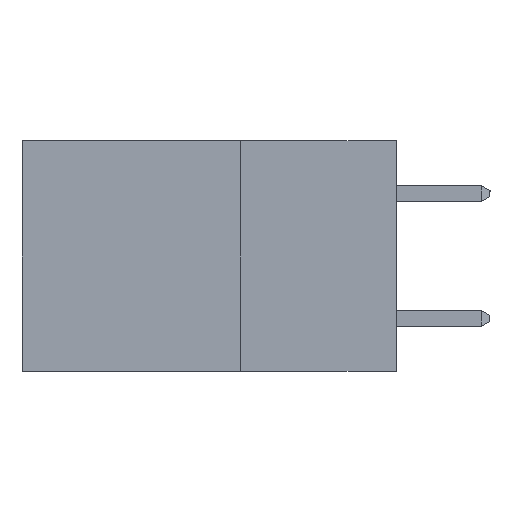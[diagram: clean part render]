
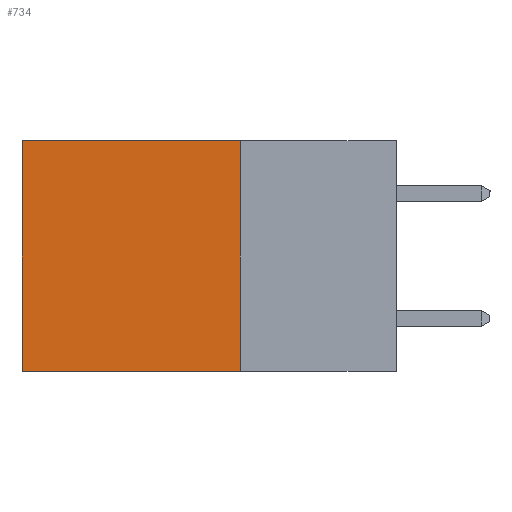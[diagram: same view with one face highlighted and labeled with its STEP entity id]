
A CAD part, left-side view. The second image highlights one B-rep face of the part: STEP entity #734.
In plain terms, the highlighted planar face has unit normal (-1, 0, 0).
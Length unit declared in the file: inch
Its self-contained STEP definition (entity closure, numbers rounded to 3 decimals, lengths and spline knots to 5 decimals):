
#233 = ORIENTED_EDGE ( 'NONE', *, *, #7456, .F. ) ;
#541 = DIRECTION ( 'NONE',  ( 1., 0., 0. ) ) ;
#602 = CARTESIAN_POINT ( 'NONE',  ( 0.2615, 0.6, -0.37 ) ) ;
#645 = CARTESIAN_POINT ( 'NONE',  ( 0.2615, 0.25, 0. ) ) ;
#662 = LINE ( 'NONE', #11323, #1744 ) ;
#734 = ADVANCED_FACE ( 'NONE', ( #12336 ), #2874, .F. ) ;
#1647 = ORIENTED_EDGE ( 'NONE', *, *, #8013, .T. ) ;
#1744 = VECTOR ( 'NONE', #6062, 39.37008 ) ;
#2865 = VECTOR ( 'NONE', #16594, 39.37008 ) ;
#2874 = PLANE ( 'NONE',  #13465 ) ;
#3467 = ORIENTED_EDGE ( 'NONE', *, *, #10542, .T. ) ;
#4374 = CARTESIAN_POINT ( 'NONE',  ( 0.2615, 0.25, -0.37 ) ) ;
#6062 = DIRECTION ( 'NONE',  ( 0., 1., 0. ) ) ;
#6127 = DIRECTION ( 'NONE',  ( 0., 0., -1. ) ) ;
#6143 = CARTESIAN_POINT ( 'NONE',  ( 0.2615, 0.6, -0.37 ) ) ;
#7348 = VERTEX_POINT ( 'NONE', #645 ) ;
#7456 = EDGE_CURVE ( 'NONE', #7348, #13316, #9012, .T. ) ;
#8013 = EDGE_CURVE ( 'NONE', #7348, #10789, #662, .T. ) ;
#8513 = LINE ( 'NONE', #6143, #2865 ) ;
#9012 = LINE ( 'NONE', #10422, #16290 ) ;
#9901 = DIRECTION ( 'NONE',  ( 0., 0., -1. ) ) ;
#10422 = CARTESIAN_POINT ( 'NONE',  ( 0.2615, 0.25, -0.37 ) ) ;
#10542 = EDGE_CURVE ( 'NONE', #10789, #15559, #8513, .T. ) ;
#10789 = VERTEX_POINT ( 'NONE', #12084 ) ;
#10847 = EDGE_LOOP ( 'NONE', ( #3467, #14903, #233, #1647 ) ) ;
#11285 = DIRECTION ( 'NONE',  ( 0., 1., 0. ) ) ;
#11323 = CARTESIAN_POINT ( 'NONE',  ( 0.2615, 0.25, 0. ) ) ;
#12084 = CARTESIAN_POINT ( 'NONE',  ( 0.2615, 0.6, 0. ) ) ;
#12336 = FACE_OUTER_BOUND ( 'NONE', #10847, .T. ) ;
#13316 = VERTEX_POINT ( 'NONE', #17204 ) ;
#13465 = AXIS2_PLACEMENT_3D ( 'NONE', #4374, #541, #9901 ) ;
#14903 = ORIENTED_EDGE ( 'NONE', *, *, #16923, .F. ) ;
#15311 = LINE ( 'NONE', #16729, #17067 ) ;
#15559 = VERTEX_POINT ( 'NONE', #602 ) ;
#16290 = VECTOR ( 'NONE', #6127, 39.37008 ) ;
#16594 = DIRECTION ( 'NONE',  ( 0., 0., -1. ) ) ;
#16729 = CARTESIAN_POINT ( 'NONE',  ( 0.2615, 0.25, -0.37 ) ) ;
#16923 = EDGE_CURVE ( 'NONE', #13316, #15559, #15311, .T. ) ;
#17067 = VECTOR ( 'NONE', #11285, 39.37008 ) ;
#17204 = CARTESIAN_POINT ( 'NONE',  ( 0.2615, 0.25, -0.37 ) ) ;
